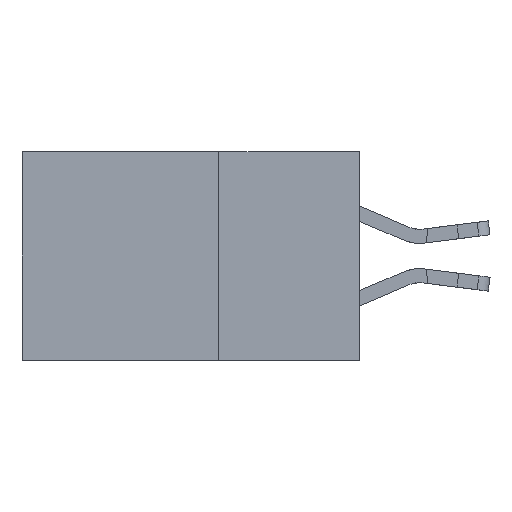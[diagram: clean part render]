
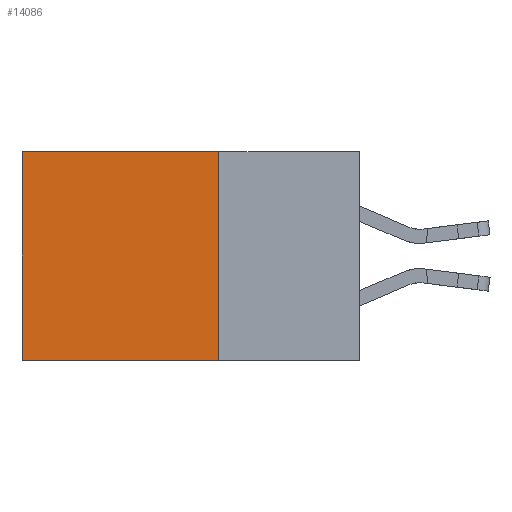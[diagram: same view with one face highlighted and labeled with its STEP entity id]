
A CAD part, left-side view. The second image highlights one B-rep face of the part: STEP entity #14086.
In plain terms, the highlighted planar face has unit normal (-1, 0, 0).
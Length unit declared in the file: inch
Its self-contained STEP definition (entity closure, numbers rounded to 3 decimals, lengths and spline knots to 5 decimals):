
#424 = DIRECTION ( 'NONE',  ( 0., 0., -1. ) ) ;
#1760 = VERTEX_POINT ( 'NONE', #10460 ) ;
#1785 = LINE ( 'NONE', #6153, #8239 ) ;
#2182 = ORIENTED_EDGE ( 'NONE', *, *, #8216, .T. ) ;
#2421 = CARTESIAN_POINT ( 'NONE',  ( 0.2875, 0.25, 0. ) ) ;
#2588 = LINE ( 'NONE', #11860, #12365 ) ;
#2960 = EDGE_LOOP ( 'NONE', ( #2182, #13742, #3995, #9380 ) ) ;
#3851 = EDGE_CURVE ( 'NONE', #14126, #4995, #8704, .T. ) ;
#3943 = EDGE_CURVE ( 'NONE', #14126, #7545, #1785, .T. ) ;
#3995 = ORIENTED_EDGE ( 'NONE', *, *, #3851, .F. ) ;
#4491 = CARTESIAN_POINT ( 'NONE',  ( 0.2875, 0.25, -0.37 ) ) ;
#4888 = VECTOR ( 'NONE', #12415, 39.37008 ) ;
#4995 = VERTEX_POINT ( 'NONE', #10037 ) ;
#5564 = DIRECTION ( 'NONE',  ( 0., 0., -1. ) ) ;
#6153 = CARTESIAN_POINT ( 'NONE',  ( 0.2875, 0.25, 0. ) ) ;
#6873 = FACE_OUTER_BOUND ( 'NONE', #2960, .T. ) ;
#7005 = DIRECTION ( 'NONE',  ( 1., 0., 0. ) ) ;
#7518 = EDGE_CURVE ( 'NONE', #4995, #1760, #15936, .T. ) ;
#7545 = VERTEX_POINT ( 'NONE', #7742 ) ;
#7742 = CARTESIAN_POINT ( 'NONE',  ( 0.2875, 0.6, 0. ) ) ;
#8216 = EDGE_CURVE ( 'NONE', #7545, #1760, #2588, .T. ) ;
#8239 = VECTOR ( 'NONE', #9032, 39.37008 ) ;
#8675 = VECTOR ( 'NONE', #17529, 39.37008 ) ;
#8704 = LINE ( 'NONE', #2421, #4888 ) ;
#9032 = DIRECTION ( 'NONE',  ( 0., 1., 0. ) ) ;
#9380 = ORIENTED_EDGE ( 'NONE', *, *, #3943, .T. ) ;
#10037 = CARTESIAN_POINT ( 'NONE',  ( 0.2875, 0.25, -0.37 ) ) ;
#10460 = CARTESIAN_POINT ( 'NONE',  ( 0.2875, 0.6, -0.37 ) ) ;
#10793 = AXIS2_PLACEMENT_3D ( 'NONE', #15683, #7005, #5564 ) ;
#11327 = CARTESIAN_POINT ( 'NONE',  ( 0.2875, 0.25, 0. ) ) ;
#11860 = CARTESIAN_POINT ( 'NONE',  ( 0.2875, 0.6, 0. ) ) ;
#12365 = VECTOR ( 'NONE', #424, 39.37008 ) ;
#12415 = DIRECTION ( 'NONE',  ( 0., 0., -1. ) ) ;
#13742 = ORIENTED_EDGE ( 'NONE', *, *, #7518, .F. ) ;
#14057 = PLANE ( 'NONE',  #10793 ) ;
#14086 = ADVANCED_FACE ( 'NONE', ( #6873 ), #14057, .F. ) ;
#14126 = VERTEX_POINT ( 'NONE', #11327 ) ;
#15683 = CARTESIAN_POINT ( 'NONE',  ( 0.2875, 0.25, 0. ) ) ;
#15936 = LINE ( 'NONE', #4491, #8675 ) ;
#17529 = DIRECTION ( 'NONE',  ( 0., 1., 0. ) ) ;
